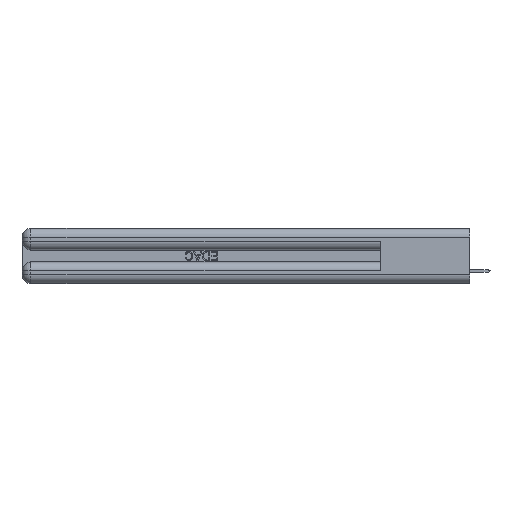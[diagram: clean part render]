
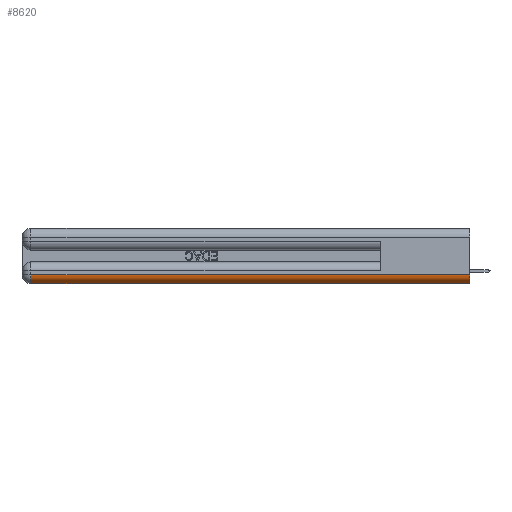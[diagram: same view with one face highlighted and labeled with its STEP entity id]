
A CAD part, left-side view. The second image highlights one B-rep face of the part: STEP entity #8620.
In plain terms, the highlighted cylindrical face has radius 1.524 mm (diameter 3.048 mm), a partial arc.
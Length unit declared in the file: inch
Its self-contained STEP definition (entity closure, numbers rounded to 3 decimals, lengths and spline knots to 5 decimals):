
#610 = AXIS2_PLACEMENT_3D ( 'NONE', #49636, #53824, #2526 ) ;
#1318 = CARTESIAN_POINT ( 'NONE',  ( 0., 0., 0.06 ) ) ;
#1661 = ORIENTED_EDGE ( 'NONE', *, *, #51441, .F. ) ;
#2526 = DIRECTION ( 'NONE',  ( 0., 0., 1. ) ) ;
#2705 = VECTOR ( 'NONE', #36038, 39.37008 ) ;
#3065 = CIRCLE ( 'NONE', #20082, 0.06 ) ;
#5039 = ORIENTED_EDGE ( 'NONE', *, *, #40879, .F. ) ;
#6803 = VERTEX_POINT ( 'NONE', #18520 ) ;
#8244 = VERTEX_POINT ( 'NONE', #16545 ) ;
#8620 = ADVANCED_FACE ( 'NONE', ( #12253 ), #46483, .T. ) ;
#10523 = EDGE_CURVE ( 'NONE', #29613, #22834, #44484, .T. ) ;
#11439 = DIRECTION ( 'NONE',  ( 0., 0., 1. ) ) ;
#12253 = FACE_OUTER_BOUND ( 'NONE', #50228, .T. ) ;
#13189 = VECTOR ( 'NONE', #34322, 39.37008 ) ;
#16545 = CARTESIAN_POINT ( 'NONE',  ( 0., 2.94, 0.06 ) ) ;
#18520 = CARTESIAN_POINT ( 'NONE',  ( 0.06, 2.94, 0. ) ) ;
#20082 = AXIS2_PLACEMENT_3D ( 'NONE', #25916, #38019, #43012 ) ;
#22834 = VERTEX_POINT ( 'NONE', #52836 ) ;
#24802 = LINE ( 'NONE', #42719, #13189 ) ;
#25916 = CARTESIAN_POINT ( 'NONE',  ( 0.06, 2.94, 0.06 ) ) ;
#29202 = ORIENTED_EDGE ( 'NONE', *, *, #48378, .F. ) ;
#29613 = VERTEX_POINT ( 'NONE', #1318 ) ;
#30746 = LINE ( 'NONE', #47828, #2705 ) ;
#34322 = DIRECTION ( 'NONE',  ( 0., 1., 0. ) ) ;
#36038 = DIRECTION ( 'NONE',  ( 0., -1., 0. ) ) ;
#38019 = DIRECTION ( 'NONE',  ( 0., 1., 0. ) ) ;
#38097 = CARTESIAN_POINT ( 'NONE',  ( 0.06, 0., 0.06 ) ) ;
#40879 = EDGE_CURVE ( 'NONE', #22834, #6803, #24802, .T. ) ;
#41381 = AXIS2_PLACEMENT_3D ( 'NONE', #38097, #46211, #11439 ) ;
#42719 = CARTESIAN_POINT ( 'NONE',  ( 0.06, 3., 0. ) ) ;
#43012 = DIRECTION ( 'NONE',  ( 0., 0., 1. ) ) ;
#44484 = CIRCLE ( 'NONE', #610, 0.06 ) ;
#46211 = DIRECTION ( 'NONE',  ( 0., 1., 0. ) ) ;
#46483 = CYLINDRICAL_SURFACE ( 'NONE', #41381, 0.06 ) ;
#47828 = CARTESIAN_POINT ( 'NONE',  ( 0., 0., 0.06 ) ) ;
#48378 = EDGE_CURVE ( 'NONE', #6803, #8244, #3065, .T. ) ;
#49636 = CARTESIAN_POINT ( 'NONE',  ( 0.06, 0., 0.06 ) ) ;
#50228 = EDGE_LOOP ( 'NONE', ( #54524, #1661, #29202, #5039 ) ) ;
#51441 = EDGE_CURVE ( 'NONE', #8244, #29613, #30746, .T. ) ;
#52836 = CARTESIAN_POINT ( 'NONE',  ( 0.06, 0., 0. ) ) ;
#53824 = DIRECTION ( 'NONE',  ( 0., -1., 0. ) ) ;
#54524 = ORIENTED_EDGE ( 'NONE', *, *, #10523, .F. ) ;
